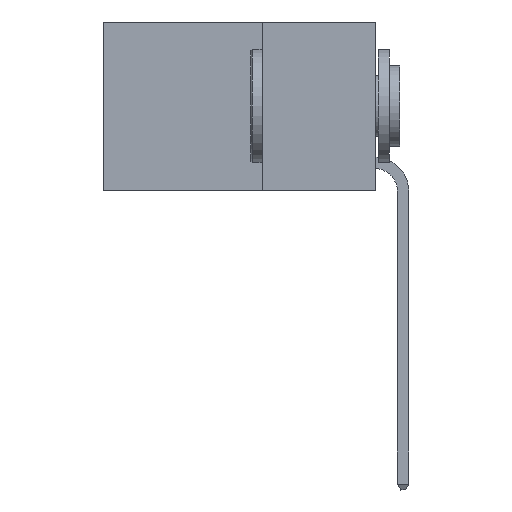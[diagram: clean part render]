
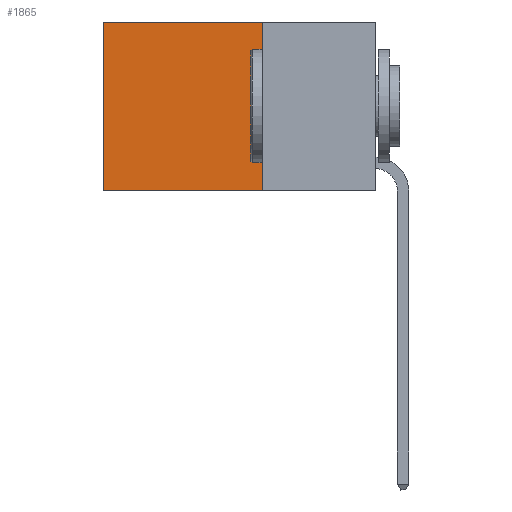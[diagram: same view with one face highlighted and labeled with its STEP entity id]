
A CAD part, left-side view. The second image highlights one B-rep face of the part: STEP entity #1865.
In plain terms, the highlighted planar face has unit normal (-1, 0, 0).
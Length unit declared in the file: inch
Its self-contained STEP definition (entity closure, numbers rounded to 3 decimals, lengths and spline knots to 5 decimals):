
#906 = VECTOR ( 'NONE', #15231, 39.37008 ) ;
#1041 = PLANE ( 'NONE',  #20745 ) ;
#1424 = VECTOR ( 'NONE', #10771, 39.37008 ) ;
#1523 = EDGE_CURVE ( 'NONE', #19283, #3074, #16219, .T. ) ;
#1823 = CARTESIAN_POINT ( 'NONE',  ( 0.2625, 0.25, -0.37 ) ) ;
#1865 = ADVANCED_FACE ( 'NONE', ( #9713 ), #1041, .F. ) ;
#3074 = VERTEX_POINT ( 'NONE', #12386 ) ;
#3278 = VECTOR ( 'NONE', #9993, 39.37008 ) ;
#4336 = CARTESIAN_POINT ( 'NONE',  ( 0.2625, 0.25, 0. ) ) ;
#5453 = EDGE_CURVE ( 'NONE', #18751, #10110, #5760, .T. ) ;
#5480 = CARTESIAN_POINT ( 'NONE',  ( 0.2625, 0.25, 0. ) ) ;
#5760 = LINE ( 'NONE', #13613, #1424 ) ;
#5935 = DIRECTION ( 'NONE',  ( 0., 0., -1. ) ) ;
#5943 = EDGE_CURVE ( 'NONE', #18751, #19283, #9046, .T. ) ;
#8692 = CARTESIAN_POINT ( 'NONE',  ( 0.2625, 0.25, -0.37 ) ) ;
#8861 = CARTESIAN_POINT ( 'NONE',  ( 0.2625, 0.25, 0. ) ) ;
#9046 = LINE ( 'NONE', #5480, #906 ) ;
#9713 = FACE_OUTER_BOUND ( 'NONE', #13041, .T. ) ;
#9889 = EDGE_CURVE ( 'NONE', #10110, #3074, #16204, .T. ) ;
#9993 = DIRECTION ( 'NONE',  ( 0., 1., 0. ) ) ;
#10110 = VERTEX_POINT ( 'NONE', #18041 ) ;
#10771 = DIRECTION ( 'NONE',  ( 0., 1., 0. ) ) ;
#12136 = ORIENTED_EDGE ( 'NONE', *, *, #5453, .T. ) ;
#12386 = CARTESIAN_POINT ( 'NONE',  ( 0.2625, 0.6, -0.37 ) ) ;
#13041 = EDGE_LOOP ( 'NONE', ( #14857, #17308, #17638, #12136 ) ) ;
#13613 = CARTESIAN_POINT ( 'NONE',  ( 0.2625, 0.25, 0. ) ) ;
#14382 = CARTESIAN_POINT ( 'NONE',  ( 0.2625, 0.6, 0. ) ) ;
#14857 = ORIENTED_EDGE ( 'NONE', *, *, #9889, .T. ) ;
#15231 = DIRECTION ( 'NONE',  ( 0., 0., -1. ) ) ;
#15683 = DIRECTION ( 'NONE',  ( 1., 0., 0. ) ) ;
#16021 = DIRECTION ( 'NONE',  ( 0., 0., -1. ) ) ;
#16204 = LINE ( 'NONE', #14382, #20449 ) ;
#16219 = LINE ( 'NONE', #1823, #3278 ) ;
#17308 = ORIENTED_EDGE ( 'NONE', *, *, #1523, .F. ) ;
#17638 = ORIENTED_EDGE ( 'NONE', *, *, #5943, .F. ) ;
#18041 = CARTESIAN_POINT ( 'NONE',  ( 0.2625, 0.6, 0. ) ) ;
#18751 = VERTEX_POINT ( 'NONE', #8861 ) ;
#19283 = VERTEX_POINT ( 'NONE', #8692 ) ;
#20449 = VECTOR ( 'NONE', #16021, 39.37008 ) ;
#20745 = AXIS2_PLACEMENT_3D ( 'NONE', #4336, #15683, #5935 ) ;
